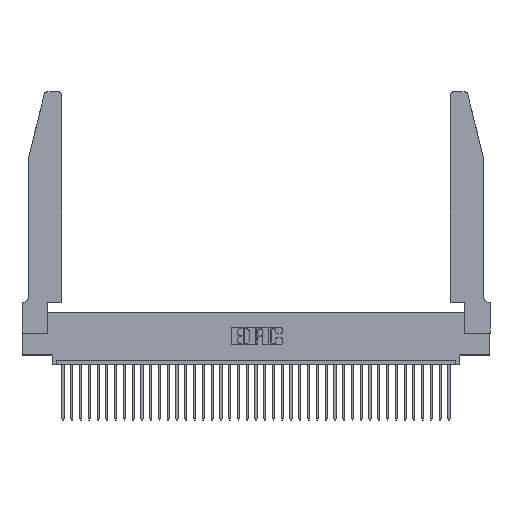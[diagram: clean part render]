
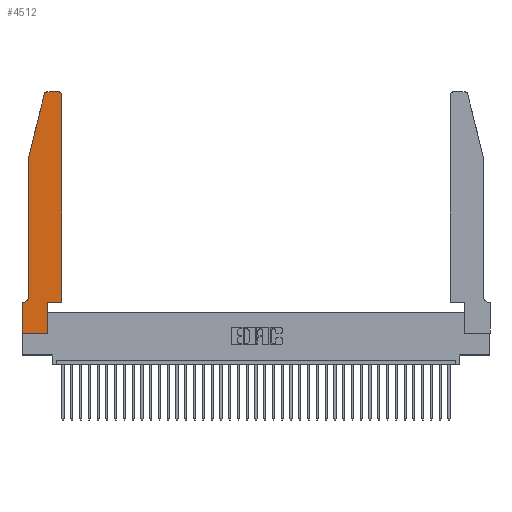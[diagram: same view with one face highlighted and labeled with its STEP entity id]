
A CAD part, top view. The second image highlights one B-rep face of the part: STEP entity #4512.
In plain terms, the highlighted planar face has unit normal (0, 0, 1).
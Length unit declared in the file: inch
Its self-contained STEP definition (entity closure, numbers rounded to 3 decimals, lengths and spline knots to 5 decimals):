
#1657 = LINE ( 'NONE', #21276, #21569 ) ;
#2289 = CIRCLE ( 'NONE', #37976, 0.03 ) ;
#2357 = LINE ( 'NONE', #18794, #31587 ) ;
#2463 = LINE ( 'NONE', #32170, #28919 ) ;
#2535 = LINE ( 'NONE', #4984, #30347 ) ;
#2737 = ORIENTED_EDGE ( 'NONE', *, *, #21294, .T. ) ;
#2948 = DIRECTION ( 'NONE',  ( 0., 1., 0. ) ) ;
#2962 = VERTEX_POINT ( 'NONE', #20507 ) ;
#3384 = ORIENTED_EDGE ( 'NONE', *, *, #10384, .T. ) ;
#3863 = CARTESIAN_POINT ( 'NONE',  ( 0.0755, 2., 0.37 ) ) ;
#4133 = AXIS2_PLACEMENT_3D ( 'NONE', #30413, #33713, #21677 ) ;
#4223 = PLANE ( 'NONE',  #19435 ) ;
#4355 = CARTESIAN_POINT ( 'NONE',  ( 0., 0.35, 0.37 ) ) ;
#4512 = ADVANCED_FACE ( 'NONE', ( #31498 ), #4223, .T. ) ;
#4882 = LINE ( 'NONE', #32304, #20586 ) ;
#4984 = CARTESIAN_POINT ( 'NONE',  ( 0.2865, 0.35, 0.37 ) ) ;
#5189 = CARTESIAN_POINT ( 'NONE',  ( 0.0755, 0.42, 0.37 ) ) ;
#5241 = ORIENTED_EDGE ( 'NONE', *, *, #29693, .T. ) ;
#5405 = EDGE_CURVE ( 'NONE', #9168, #7357, #2463, .T. ) ;
#6610 = DIRECTION ( 'NONE',  ( 0., -1., 0. ) ) ;
#7124 = EDGE_CURVE ( 'NONE', #34766, #24819, #8290, .T. ) ;
#7357 = VERTEX_POINT ( 'NONE', #31762 ) ;
#7515 = VERTEX_POINT ( 'NONE', #35148 ) ;
#7812 = DIRECTION ( 'NONE',  ( 0., 0., 1. ) ) ;
#8290 = CIRCLE ( 'NONE', #4133, 0.07 ) ;
#9123 = EDGE_CURVE ( 'NONE', #24819, #2962, #1657, .T. ) ;
#9168 = VERTEX_POINT ( 'NONE', #12110 ) ;
#9196 = VERTEX_POINT ( 'NONE', #35698 ) ;
#9319 = CIRCLE ( 'NONE', #25658, 0.03 ) ;
#10367 = CARTESIAN_POINT ( 'NONE',  ( 0.0055, 0.35, 0.37 ) ) ;
#10384 = EDGE_CURVE ( 'NONE', #2962, #9196, #11304, .T. ) ;
#10618 = DIRECTION ( 'NONE',  ( 0., 0., 1. ) ) ;
#10869 = DIRECTION ( 'NONE',  ( 1., 0., 0. ) ) ;
#10943 = ORIENTED_EDGE ( 'NONE', *, *, #19411, .T. ) ;
#11304 = LINE ( 'NONE', #14222, #34514 ) ;
#12110 = CARTESIAN_POINT ( 'NONE',  ( 0.4205, 2.75, 0.37 ) ) ;
#12163 = CARTESIAN_POINT ( 'NONE',  ( 0.25487, 2.72718, 0.37 ) ) ;
#12354 = LINE ( 'NONE', #29551, #27276 ) ;
#12533 = DIRECTION ( 'NONE',  ( -1., 0., 0. ) ) ;
#12549 = EDGE_CURVE ( 'NONE', #7357, #35674, #2289, .T. ) ;
#12888 = ORIENTED_EDGE ( 'NONE', *, *, #27781, .T. ) ;
#13345 = DIRECTION ( 'NONE',  ( 1., 0., 0. ) ) ;
#13442 = VECTOR ( 'NONE', #18434, 39.37008 ) ;
#14222 = CARTESIAN_POINT ( 'NONE',  ( 0., 0., 0.37 ) ) ;
#15086 = CARTESIAN_POINT ( 'NONE',  ( 0.4505, 0.35, 0.37 ) ) ;
#15587 = CARTESIAN_POINT ( 'NONE',  ( 0.0755, 2., 0.37 ) ) ;
#16341 = CARTESIAN_POINT ( 'NONE',  ( 0.4205, 2.72, 0.37 ) ) ;
#17399 = VERTEX_POINT ( 'NONE', #27257 ) ;
#17662 = VERTEX_POINT ( 'NONE', #22484 ) ;
#18434 = DIRECTION ( 'NONE',  ( -0.239, -0.971, 0. ) ) ;
#18794 = CARTESIAN_POINT ( 'NONE',  ( 0.0755, 2., 0.37 ) ) ;
#19411 = EDGE_CURVE ( 'NONE', #17662, #17399, #4882, .T. ) ;
#19435 = AXIS2_PLACEMENT_3D ( 'NONE', #4355, #7812, #13345 ) ;
#20343 = DIRECTION ( 'NONE',  ( -1., 0., 0. ) ) ;
#20507 = CARTESIAN_POINT ( 'NONE',  ( 0., 0.35, 0.37 ) ) ;
#20523 = EDGE_CURVE ( 'NONE', #7515, #9168, #9319, .T. ) ;
#20586 = VECTOR ( 'NONE', #30991, 39.37008 ) ;
#21276 = CARTESIAN_POINT ( 'NONE',  ( 0.0755, 0.35, 0.37 ) ) ;
#21294 = EDGE_CURVE ( 'NONE', #17399, #7515, #32504, .T. ) ;
#21376 = EDGE_CURVE ( 'NONE', #35674, #28954, #29314, .T. ) ;
#21569 = VECTOR ( 'NONE', #12533, 39.37008 ) ;
#21677 = DIRECTION ( 'NONE',  ( -1., 0., 0. ) ) ;
#21934 = VERTEX_POINT ( 'NONE', #32734 ) ;
#22123 = ORIENTED_EDGE ( 'NONE', *, *, #20523, .T. ) ;
#22348 = DIRECTION ( 'NONE',  ( 0., 1., 0. ) ) ;
#22399 = ORIENTED_EDGE ( 'NONE', *, *, #5405, .T. ) ;
#22484 = CARTESIAN_POINT ( 'NONE',  ( 0.2865, 0.35, 0.37 ) ) ;
#22591 = DIRECTION ( 'NONE',  ( 0., 0., 1. ) ) ;
#22718 = DIRECTION ( 'NONE',  ( 1., 0., 0. ) ) ;
#23952 = DIRECTION ( 'NONE',  ( 1., 0., 0. ) ) ;
#24819 = VERTEX_POINT ( 'NONE', #10367 ) ;
#25658 = AXIS2_PLACEMENT_3D ( 'NONE', #16341, #10618, #10869 ) ;
#25951 = CARTESIAN_POINT ( 'NONE',  ( 0.284, 2.72, 0.37 ) ) ;
#26874 = ORIENTED_EDGE ( 'NONE', *, *, #21376, .T. ) ;
#27257 = CARTESIAN_POINT ( 'NONE',  ( 0.4505, 0.35, 0.37 ) ) ;
#27276 = VECTOR ( 'NONE', #23952, 39.37008 ) ;
#27781 = EDGE_CURVE ( 'NONE', #9196, #21934, #12354, .T. ) ;
#28048 = DIRECTION ( 'NONE',  ( 0., -1., 0. ) ) ;
#28919 = VECTOR ( 'NONE', #20343, 39.37008 ) ;
#28954 = VERTEX_POINT ( 'NONE', #3863 ) ;
#29314 = LINE ( 'NONE', #15587, #13442 ) ;
#29551 = CARTESIAN_POINT ( 'NONE',  ( 0., 0., 0.37 ) ) ;
#29693 = EDGE_CURVE ( 'NONE', #21934, #17662, #2535, .T. ) ;
#29720 = ORIENTED_EDGE ( 'NONE', *, *, #7124, .T. ) ;
#30313 = EDGE_LOOP ( 'NONE', ( #22399, #36562, #26874, #33557, #29720, #36680, #3384, #12888, #5241, #10943, #2737, #22123 ) ) ;
#30347 = VECTOR ( 'NONE', #22348, 39.37008 ) ;
#30413 = CARTESIAN_POINT ( 'NONE',  ( 0.0055, 0.42, 0.37 ) ) ;
#30991 = DIRECTION ( 'NONE',  ( 1., 0., 0. ) ) ;
#31498 = FACE_OUTER_BOUND ( 'NONE', #30313, .T. ) ;
#31587 = VECTOR ( 'NONE', #28048, 39.37008 ) ;
#31668 = EDGE_CURVE ( 'NONE', #28954, #34766, #2357, .T. ) ;
#31762 = CARTESIAN_POINT ( 'NONE',  ( 0.284, 2.75, 0.37 ) ) ;
#32170 = CARTESIAN_POINT ( 'NONE',  ( 0.2605, 2.75, 0.37 ) ) ;
#32304 = CARTESIAN_POINT ( 'NONE',  ( 0.4505, 0.35, 0.37 ) ) ;
#32504 = LINE ( 'NONE', #15086, #35263 ) ;
#32734 = CARTESIAN_POINT ( 'NONE',  ( 0.2865, 0., 0.37 ) ) ;
#33557 = ORIENTED_EDGE ( 'NONE', *, *, #31668, .T. ) ;
#33713 = DIRECTION ( 'NONE',  ( 0., 0., -1. ) ) ;
#34514 = VECTOR ( 'NONE', #6610, 39.37008 ) ;
#34766 = VERTEX_POINT ( 'NONE', #5189 ) ;
#35148 = CARTESIAN_POINT ( 'NONE',  ( 0.4505, 2.72, 0.37 ) ) ;
#35263 = VECTOR ( 'NONE', #2948, 39.37008 ) ;
#35674 = VERTEX_POINT ( 'NONE', #12163 ) ;
#35698 = CARTESIAN_POINT ( 'NONE',  ( 0., 0., 0.37 ) ) ;
#36562 = ORIENTED_EDGE ( 'NONE', *, *, #12549, .T. ) ;
#36680 = ORIENTED_EDGE ( 'NONE', *, *, #9123, .T. ) ;
#37976 = AXIS2_PLACEMENT_3D ( 'NONE', #25951, #22591, #22718 ) ;
